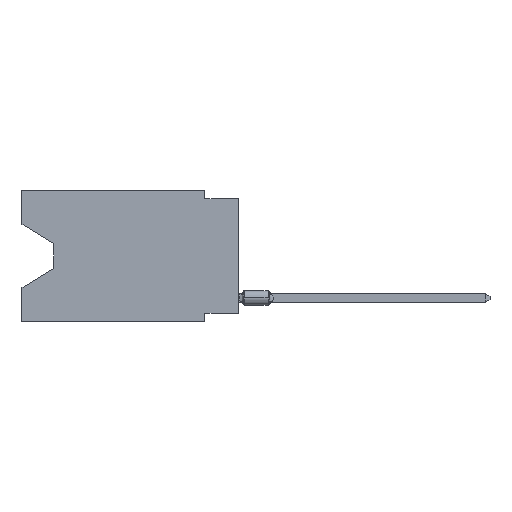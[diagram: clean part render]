
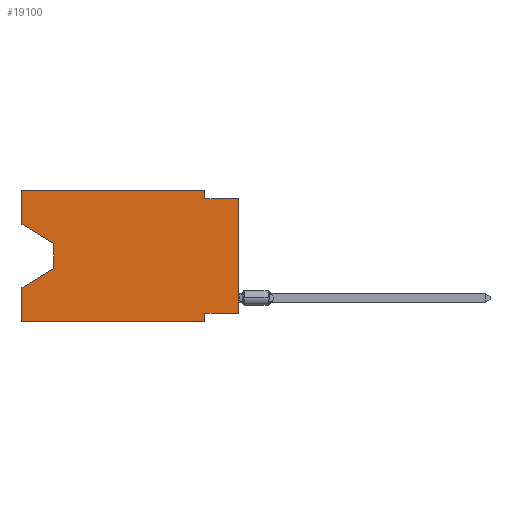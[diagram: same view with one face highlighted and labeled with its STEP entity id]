
A CAD part, left-side view. The second image highlights one B-rep face of the part: STEP entity #19100.
In plain terms, the highlighted planar face has unit normal (-1, 0, 0).
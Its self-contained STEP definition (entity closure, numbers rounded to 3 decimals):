
#11 = CARTESIAN_POINT ( 'NONE',  ( 0., 0., -9.271 ) ) ;
#14 = VERTEX_POINT ( 'NONE', #12429 ) ;
#53 = VECTOR ( 'NONE', #15855, 1000. ) ;
#65 = VERTEX_POINT ( 'NONE', #7749 ) ;
#511 = EDGE_CURVE ( 'NONE', #4172, #10413, #8956, .T. ) ;
#583 = EDGE_LOOP ( 'NONE', ( #3444, #3119, #14497, #15684, #19009, #7704, #16788, #9534, #13939, #18567, #1081, #9911 ) ) ;
#768 = PLANE ( 'NONE',  #18337 ) ;
#1066 = EDGE_CURVE ( 'NONE', #12320, #14083, #2042, .T. ) ;
#1081 = ORIENTED_EDGE ( 'NONE', *, *, #15491, .F. ) ;
#1159 = VERTEX_POINT ( 'NONE', #16345 ) ;
#1544 = CARTESIAN_POINT ( 'NONE',  ( 0., 13.97, -5.893 ) ) ;
#1681 = DIRECTION ( 'NONE',  ( 0., -1., 0. ) ) ;
#1849 = EDGE_CURVE ( 'NONE', #12320, #6480, #3788, .T. ) ;
#2042 = LINE ( 'NONE', #15765, #53 ) ;
#2064 = DIRECTION ( 'NONE',  ( 0., 0., -1. ) ) ;
#2155 = VERTEX_POINT ( 'NONE', #18363 ) ;
#2187 = CARTESIAN_POINT ( 'NONE',  ( 0., 16.383, -9.906 ) ) ;
#2302 = VECTOR ( 'NONE', #1681, 1000. ) ;
#2634 = CARTESIAN_POINT ( 'NONE',  ( 0., 13.97, -4.013 ) ) ;
#3042 = DIRECTION ( 'NONE',  ( 0., 0.855, -0.519 ) ) ;
#3119 = ORIENTED_EDGE ( 'NONE', *, *, #14015, .T. ) ;
#3140 = DIRECTION ( 'NONE',  ( 0., -1., 0. ) ) ;
#3168 = CARTESIAN_POINT ( 'NONE',  ( 0., 0., -0.635 ) ) ;
#3370 = CARTESIAN_POINT ( 'NONE',  ( 0., 13.97, -4.013 ) ) ;
#3444 = ORIENTED_EDGE ( 'NONE', *, *, #511, .T. ) ;
#3788 = LINE ( 'NONE', #6665, #14998 ) ;
#4172 = VERTEX_POINT ( 'NONE', #9287 ) ;
#4347 = LINE ( 'NONE', #9022, #7148 ) ;
#4724 = CARTESIAN_POINT ( 'NONE',  ( 0., 2.54, -9.906 ) ) ;
#4749 = EDGE_CURVE ( 'NONE', #13448, #65, #5202, .T. ) ;
#5145 = VECTOR ( 'NONE', #18295, 1000. ) ;
#5202 = LINE ( 'NONE', #7882, #14291 ) ;
#5257 = CARTESIAN_POINT ( 'NONE',  ( 0., 16.383, -7.36 ) ) ;
#5415 = VECTOR ( 'NONE', #6227, 1000. ) ;
#5706 = LINE ( 'NONE', #9087, #12461 ) ;
#5713 = CARTESIAN_POINT ( 'NONE',  ( 0., 16.383, 0. ) ) ;
#5902 = DIRECTION ( 'NONE',  ( 0., 0., 1. ) ) ;
#6227 = DIRECTION ( 'NONE',  ( 0., 0., -1. ) ) ;
#6480 = VERTEX_POINT ( 'NONE', #10059 ) ;
#6665 = CARTESIAN_POINT ( 'NONE',  ( 0., 16.383, -9.906 ) ) ;
#6726 = VERTEX_POINT ( 'NONE', #8146 ) ;
#6826 = DIRECTION ( 'NONE',  ( 0., 0., -1. ) ) ;
#7147 = EDGE_CURVE ( 'NONE', #65, #6480, #14184, .T. ) ;
#7148 = VECTOR ( 'NONE', #3140, 1000. ) ;
#7425 = LINE ( 'NONE', #1544, #8432 ) ;
#7704 = ORIENTED_EDGE ( 'NONE', *, *, #7147, .F. ) ;
#7749 = CARTESIAN_POINT ( 'NONE',  ( 0., 2.54, -9.271 ) ) ;
#7882 = CARTESIAN_POINT ( 'NONE',  ( 0., 0., -9.271 ) ) ;
#8146 = CARTESIAN_POINT ( 'NONE',  ( 0., 13.97, -5.893 ) ) ;
#8182 = EDGE_CURVE ( 'NONE', #13448, #2155, #5706, .T. ) ;
#8224 = CARTESIAN_POINT ( 'NONE',  ( 0., 2.54, 0. ) ) ;
#8432 = VECTOR ( 'NONE', #3042, 1000. ) ;
#8642 = EDGE_CURVE ( 'NONE', #1159, #2155, #12335, .T. ) ;
#8956 = LINE ( 'NONE', #12250, #5145 ) ;
#9022 = CARTESIAN_POINT ( 'NONE',  ( 0., 16.383, 0. ) ) ;
#9087 = CARTESIAN_POINT ( 'NONE',  ( 0., 0., 0. ) ) ;
#9287 = CARTESIAN_POINT ( 'NONE',  ( 0., 16.383, -2.546 ) ) ;
#9534 = ORIENTED_EDGE ( 'NONE', *, *, #8182, .T. ) ;
#9911 = ORIENTED_EDGE ( 'NONE', *, *, #15805, .F. ) ;
#9959 = VECTOR ( 'NONE', #6826, 1000. ) ;
#10059 = CARTESIAN_POINT ( 'NONE',  ( 0., 2.54, -9.906 ) ) ;
#10413 = VERTEX_POINT ( 'NONE', #2634 ) ;
#11104 = LINE ( 'NONE', #8224, #9959 ) ;
#11414 = FACE_OUTER_BOUND ( 'NONE', #583, .T. ) ;
#11703 = DIRECTION ( 'NONE',  ( 0., 0., 1. ) ) ;
#11777 = CARTESIAN_POINT ( 'NONE',  ( 0., 2.54, 0. ) ) ;
#12225 = DIRECTION ( 'NONE',  ( 0., 0., -1. ) ) ;
#12249 = VECTOR ( 'NONE', #11703, 1000. ) ;
#12250 = CARTESIAN_POINT ( 'NONE',  ( 0., 16.383, -2.546 ) ) ;
#12320 = VERTEX_POINT ( 'NONE', #2187 ) ;
#12335 = LINE ( 'NONE', #3168, #2302 ) ;
#12429 = CARTESIAN_POINT ( 'NONE',  ( 0., 16.383, 0. ) ) ;
#12461 = VECTOR ( 'NONE', #5902, 1000. ) ;
#12473 = DIRECTION ( 'NONE',  ( 0., 1., 0. ) ) ;
#13274 = VERTEX_POINT ( 'NONE', #11777 ) ;
#13448 = VERTEX_POINT ( 'NONE', #11 ) ;
#13939 = ORIENTED_EDGE ( 'NONE', *, *, #8642, .F. ) ;
#14015 = EDGE_CURVE ( 'NONE', #10413, #6726, #16986, .T. ) ;
#14083 = VERTEX_POINT ( 'NONE', #5257 ) ;
#14184 = LINE ( 'NONE', #4724, #5415 ) ;
#14291 = VECTOR ( 'NONE', #12473, 1000. ) ;
#14497 = ORIENTED_EDGE ( 'NONE', *, *, #16140, .T. ) ;
#14538 = EDGE_CURVE ( 'NONE', #13274, #1159, #11104, .T. ) ;
#14998 = VECTOR ( 'NONE', #17506, 1000. ) ;
#15491 = EDGE_CURVE ( 'NONE', #14, #13274, #4347, .T. ) ;
#15584 = DIRECTION ( 'NONE',  ( 1., 0., 0. ) ) ;
#15684 = ORIENTED_EDGE ( 'NONE', *, *, #1066, .F. ) ;
#15765 = CARTESIAN_POINT ( 'NONE',  ( 0., 16.383, 0. ) ) ;
#15805 = EDGE_CURVE ( 'NONE', #4172, #14, #19247, .T. ) ;
#15855 = DIRECTION ( 'NONE',  ( 0., 0., 1. ) ) ;
#16042 = VECTOR ( 'NONE', #12225, 1000. ) ;
#16140 = EDGE_CURVE ( 'NONE', #6726, #14083, #7425, .T. ) ;
#16345 = CARTESIAN_POINT ( 'NONE',  ( 0., 2.54, -0.635 ) ) ;
#16788 = ORIENTED_EDGE ( 'NONE', *, *, #4749, .F. ) ;
#16986 = LINE ( 'NONE', #3370, #16042 ) ;
#17506 = DIRECTION ( 'NONE',  ( 0., -1., 0. ) ) ;
#18295 = DIRECTION ( 'NONE',  ( 0., -0.855, -0.519 ) ) ;
#18337 = AXIS2_PLACEMENT_3D ( 'NONE', #18657, #15584, #2064 ) ;
#18363 = CARTESIAN_POINT ( 'NONE',  ( 0., 0., -0.635 ) ) ;
#18567 = ORIENTED_EDGE ( 'NONE', *, *, #14538, .F. ) ;
#18657 = CARTESIAN_POINT ( 'NONE',  ( 0., 16.383, 0. ) ) ;
#19009 = ORIENTED_EDGE ( 'NONE', *, *, #1849, .T. ) ;
#19100 = ADVANCED_FACE ( 'NONE', ( #11414 ), #768, .F. ) ;
#19247 = LINE ( 'NONE', #5713, #12249 ) ;
